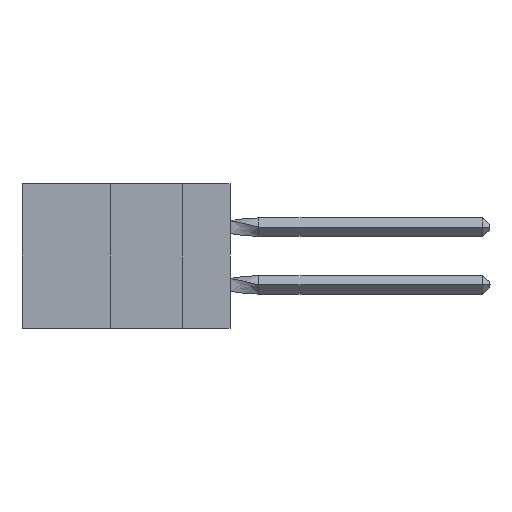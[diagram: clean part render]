
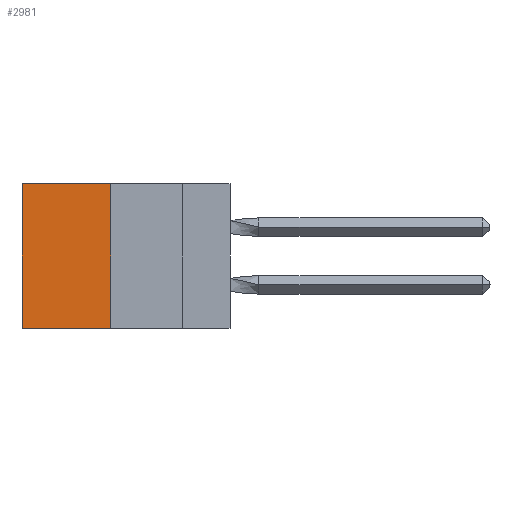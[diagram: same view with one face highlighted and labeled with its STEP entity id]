
A CAD part, left-side view. The second image highlights one B-rep face of the part: STEP entity #2981.
In plain terms, the highlighted planar face has unit normal (-1, 0, 0).
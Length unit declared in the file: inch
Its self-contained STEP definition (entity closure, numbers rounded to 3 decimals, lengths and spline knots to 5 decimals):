
#2931 = DIRECTION ( 'NONE',  ( 0., 1., 0. ) ) ;
#2937 = CARTESIAN_POINT ( 'NONE',  ( 0.305, 0.72, -0.5 ) ) ;
#2981 = ADVANCED_FACE ( 'NONE', ( #39078 ), #31755, .F. ) ;
#3553 = VECTOR ( 'NONE', #13493, 39.37008 ) ;
#5390 = EDGE_CURVE ( 'NONE', #15824, #34395, #28455, .T. ) ;
#5433 = ORIENTED_EDGE ( 'NONE', *, *, #12176, .F. ) ;
#6590 = LINE ( 'NONE', #12298, #31531 ) ;
#10879 = VERTEX_POINT ( 'NONE', #21639 ) ;
#11183 = CARTESIAN_POINT ( 'NONE',  ( 0.305, 0.413, -0.5 ) ) ;
#11779 = ORIENTED_EDGE ( 'NONE', *, *, #5390, .F. ) ;
#12176 = EDGE_CURVE ( 'NONE', #34395, #35147, #13875, .T. ) ;
#12298 = CARTESIAN_POINT ( 'NONE',  ( 0.305, 0.413, 0. ) ) ;
#12992 = DIRECTION ( 'NONE',  ( 1., 0., 0. ) ) ;
#13298 = EDGE_CURVE ( 'NONE', #15824, #10879, #6590, .T. ) ;
#13493 = DIRECTION ( 'NONE',  ( 0., 0., -1. ) ) ;
#13875 = LINE ( 'NONE', #27375, #28300 ) ;
#14982 = VECTOR ( 'NONE', #20459, 39.37008 ) ;
#15824 = VERTEX_POINT ( 'NONE', #28211 ) ;
#18700 = AXIS2_PLACEMENT_3D ( 'NONE', #34502, #12992, #22118 ) ;
#19307 = EDGE_LOOP ( 'NONE', ( #20404, #5433, #11779, #24252 ) ) ;
#19490 = EDGE_CURVE ( 'NONE', #10879, #35147, #36743, .T. ) ;
#20404 = ORIENTED_EDGE ( 'NONE', *, *, #19490, .T. ) ;
#20459 = DIRECTION ( 'NONE',  ( 0., 0., -1. ) ) ;
#21639 = CARTESIAN_POINT ( 'NONE',  ( 0.305, 0.72, 0. ) ) ;
#21819 = DIRECTION ( 'NONE',  ( 0., 1., 0. ) ) ;
#22118 = DIRECTION ( 'NONE',  ( 0., 0., -1. ) ) ;
#24252 = ORIENTED_EDGE ( 'NONE', *, *, #13298, .T. ) ;
#27375 = CARTESIAN_POINT ( 'NONE',  ( 0.305, 0.413, -0.5 ) ) ;
#28211 = CARTESIAN_POINT ( 'NONE',  ( 0.305, 0.413, 0. ) ) ;
#28300 = VECTOR ( 'NONE', #2931, 39.37008 ) ;
#28455 = LINE ( 'NONE', #36216, #14982 ) ;
#31531 = VECTOR ( 'NONE', #21819, 39.37008 ) ;
#31755 = PLANE ( 'NONE',  #18700 ) ;
#31855 = CARTESIAN_POINT ( 'NONE',  ( 0.305, 0.72, -0.5 ) ) ;
#34395 = VERTEX_POINT ( 'NONE', #11183 ) ;
#34502 = CARTESIAN_POINT ( 'NONE',  ( 0.305, 0.413, -0.5 ) ) ;
#35147 = VERTEX_POINT ( 'NONE', #2937 ) ;
#36216 = CARTESIAN_POINT ( 'NONE',  ( 0.305, 0.413, -0.5 ) ) ;
#36743 = LINE ( 'NONE', #31855, #3553 ) ;
#39078 = FACE_OUTER_BOUND ( 'NONE', #19307, .T. ) ;
